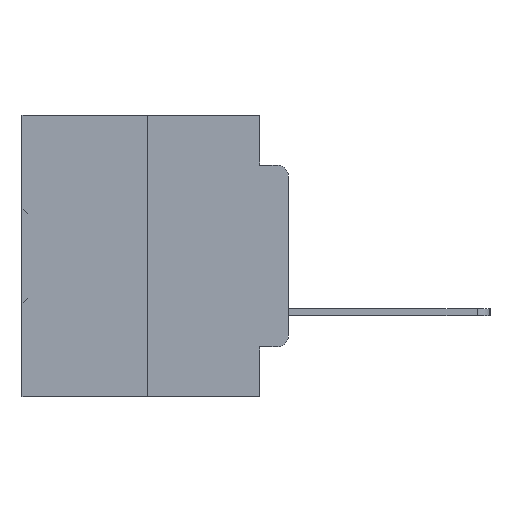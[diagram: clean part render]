
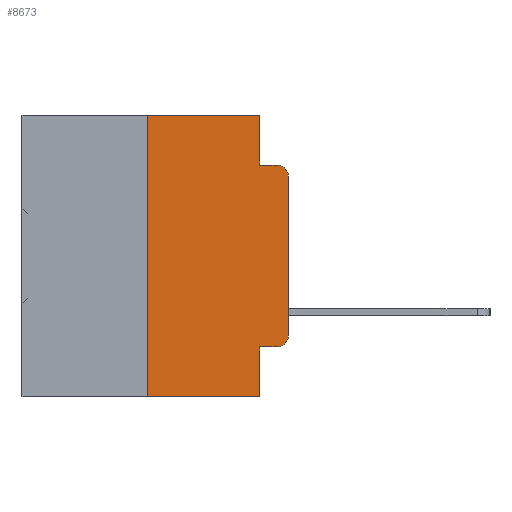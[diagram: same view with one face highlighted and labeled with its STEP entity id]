
A CAD part, left-side view. The second image highlights one B-rep face of the part: STEP entity #8673.
In plain terms, the highlighted planar face has unit normal (-1, 0, 0).
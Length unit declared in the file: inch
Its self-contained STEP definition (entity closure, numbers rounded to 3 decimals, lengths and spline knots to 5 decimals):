
#318 = EDGE_LOOP ( 'NONE', ( #6997, #19388, #14581, #11397, #12068, #15827, #17136, #24062, #28350, #6938 ) ) ;
#1131 = VERTEX_POINT ( 'NONE', #8494 ) ;
#1800 = LINE ( 'NONE', #2548, #23537 ) ;
#1827 = DIRECTION ( 'NONE',  ( 0., 0., -1. ) ) ;
#2548 = CARTESIAN_POINT ( 'NONE',  ( 0., 0.051, 0. ) ) ;
#2625 = LINE ( 'NONE', #21811, #16897 ) ;
#3694 = CARTESIAN_POINT ( 'NONE',  ( 0., 0.051, -0.5 ) ) ;
#5453 = DIRECTION ( 'NONE',  ( 0., 0., -1. ) ) ;
#5553 = CARTESIAN_POINT ( 'NONE',  ( 0., 0.02, -0.0885 ) ) ;
#6921 = DIRECTION ( 'NONE',  ( 0., 0., -1. ) ) ;
#6938 = ORIENTED_EDGE ( 'NONE', *, *, #35642, .T. ) ;
#6997 = ORIENTED_EDGE ( 'NONE', *, *, #14605, .T. ) ;
#7409 = VERTEX_POINT ( 'NONE', #3694 ) ;
#7672 = LINE ( 'NONE', #35550, #21761 ) ;
#8138 = DIRECTION ( 'NONE',  ( -1., 0., 0. ) ) ;
#8325 = EDGE_CURVE ( 'NONE', #1131, #7409, #18430, .T. ) ;
#8494 = CARTESIAN_POINT ( 'NONE',  ( 0., 0.25, -0.5 ) ) ;
#8673 = ADVANCED_FACE ( 'NONE', ( #21009 ), #20966, .F. ) ;
#8843 = CARTESIAN_POINT ( 'NONE',  ( 0., 0.473, 0. ) ) ;
#9618 = CARTESIAN_POINT ( 'NONE',  ( 0., 0.25, 0. ) ) ;
#9683 = AXIS2_PLACEMENT_3D ( 'NONE', #15238, #23786, #6921 ) ;
#10082 = CARTESIAN_POINT ( 'NONE',  ( 0., 0.02, -0.3915 ) ) ;
#10537 = VECTOR ( 'NONE', #10710, 39.37008 ) ;
#10710 = DIRECTION ( 'NONE',  ( 0., -1., 0. ) ) ;
#11397 = ORIENTED_EDGE ( 'NONE', *, *, #24919, .F. ) ;
#11433 = LINE ( 'NONE', #24709, #10537 ) ;
#11825 = EDGE_CURVE ( 'NONE', #20516, #36343, #13317, .T. ) ;
#12068 = ORIENTED_EDGE ( 'NONE', *, *, #11825, .F. ) ;
#12476 = DIRECTION ( 'NONE',  ( 0., 0., 1. ) ) ;
#12931 = DIRECTION ( 'NONE',  ( 0., 0., -1. ) ) ;
#13007 = EDGE_CURVE ( 'NONE', #1131, #20516, #36011, .T. ) ;
#13229 = LINE ( 'NONE', #17435, #14130 ) ;
#13317 = LINE ( 'NONE', #8843, #25561 ) ;
#13803 = VECTOR ( 'NONE', #12476, 39.37008 ) ;
#14130 = VECTOR ( 'NONE', #17310, 39.37008 ) ;
#14581 = ORIENTED_EDGE ( 'NONE', *, *, #18193, .F. ) ;
#14605 = EDGE_CURVE ( 'NONE', #32764, #23311, #13229, .T. ) ;
#14974 = VERTEX_POINT ( 'NONE', #31599 ) ;
#15238 = CARTESIAN_POINT ( 'NONE',  ( 0., 0.473, 0. ) ) ;
#15827 = ORIENTED_EDGE ( 'NONE', *, *, #13007, .F. ) ;
#16097 = CARTESIAN_POINT ( 'NONE',  ( 0., 0.473, -0.5 ) ) ;
#16278 = VERTEX_POINT ( 'NONE', #26655 ) ;
#16897 = VECTOR ( 'NONE', #35662, 39.37008 ) ;
#17013 = CIRCLE ( 'NONE', #20535, 0.02 ) ;
#17136 = ORIENTED_EDGE ( 'NONE', *, *, #8325, .T. ) ;
#17310 = DIRECTION ( 'NONE',  ( 0., 0., 1. ) ) ;
#17435 = CARTESIAN_POINT ( 'NONE',  ( 0., 0., 0. ) ) ;
#18193 = EDGE_CURVE ( 'NONE', #34939, #35903, #2625, .T. ) ;
#18430 = LINE ( 'NONE', #16097, #24960 ) ;
#18920 = CARTESIAN_POINT ( 'NONE',  ( 0., 0.051, 0. ) ) ;
#19388 = ORIENTED_EDGE ( 'NONE', *, *, #29417, .T. ) ;
#20180 = DIRECTION ( 'NONE',  ( 0., -1., 0. ) ) ;
#20516 = VERTEX_POINT ( 'NONE', #34057 ) ;
#20535 = AXIS2_PLACEMENT_3D ( 'NONE', #24961, #8138, #27775 ) ;
#20966 = PLANE ( 'NONE',  #9683 ) ;
#21009 = FACE_OUTER_BOUND ( 'NONE', #318, .T. ) ;
#21710 = DIRECTION ( 'NONE',  ( 0., -1., 0. ) ) ;
#21761 = VECTOR ( 'NONE', #1827, 39.37008 ) ;
#21811 = CARTESIAN_POINT ( 'NONE',  ( 0., 0.051, -0.0885 ) ) ;
#22129 = CARTESIAN_POINT ( 'NONE',  ( 0., 0., -0.3915 ) ) ;
#23311 = VERTEX_POINT ( 'NONE', #28017 ) ;
#23537 = VECTOR ( 'NONE', #5453, 39.37008 ) ;
#23786 = DIRECTION ( 'NONE',  ( 1., 0., 0. ) ) ;
#24062 = ORIENTED_EDGE ( 'NONE', *, *, #34553, .F. ) ;
#24709 = CARTESIAN_POINT ( 'NONE',  ( 0., 0.051, -0.4115 ) ) ;
#24919 = EDGE_CURVE ( 'NONE', #36343, #34939, #7672, .T. ) ;
#24960 = VECTOR ( 'NONE', #21710, 39.37008 ) ;
#24961 = CARTESIAN_POINT ( 'NONE',  ( 0., 0.02, -0.1085 ) ) ;
#25561 = VECTOR ( 'NONE', #20180, 39.37008 ) ;
#26655 = CARTESIAN_POINT ( 'NONE',  ( 0., 0.051, -0.4115 ) ) ;
#27775 = DIRECTION ( 'NONE',  ( 0., 0., -1. ) ) ;
#28017 = CARTESIAN_POINT ( 'NONE',  ( 0., 0., -0.1085 ) ) ;
#28350 = ORIENTED_EDGE ( 'NONE', *, *, #31245, .T. ) ;
#29417 = EDGE_CURVE ( 'NONE', #23311, #35903, #17013, .T. ) ;
#29707 = DIRECTION ( 'NONE',  ( -1., 0., 0. ) ) ;
#31245 = EDGE_CURVE ( 'NONE', #16278, #14974, #11433, .T. ) ;
#31599 = CARTESIAN_POINT ( 'NONE',  ( 0., 0.02, -0.4115 ) ) ;
#32179 = CIRCLE ( 'NONE', #35144, 0.02 ) ;
#32764 = VERTEX_POINT ( 'NONE', #22129 ) ;
#33982 = CARTESIAN_POINT ( 'NONE',  ( 0., 0.051, -0.0885 ) ) ;
#34057 = CARTESIAN_POINT ( 'NONE',  ( 0., 0.25, 0. ) ) ;
#34553 = EDGE_CURVE ( 'NONE', #16278, #7409, #1800, .T. ) ;
#34939 = VERTEX_POINT ( 'NONE', #33982 ) ;
#35144 = AXIS2_PLACEMENT_3D ( 'NONE', #10082, #29707, #12931 ) ;
#35550 = CARTESIAN_POINT ( 'NONE',  ( 0., 0.051, 0. ) ) ;
#35642 = EDGE_CURVE ( 'NONE', #14974, #32764, #32179, .T. ) ;
#35662 = DIRECTION ( 'NONE',  ( 0., -1., 0. ) ) ;
#35903 = VERTEX_POINT ( 'NONE', #5553 ) ;
#36011 = LINE ( 'NONE', #9618, #13803 ) ;
#36343 = VERTEX_POINT ( 'NONE', #18920 ) ;
